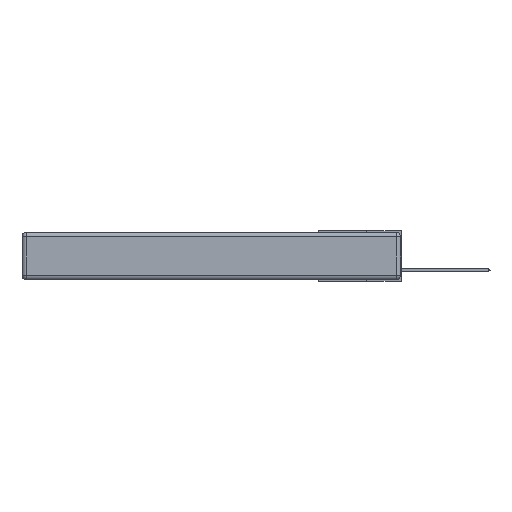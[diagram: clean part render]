
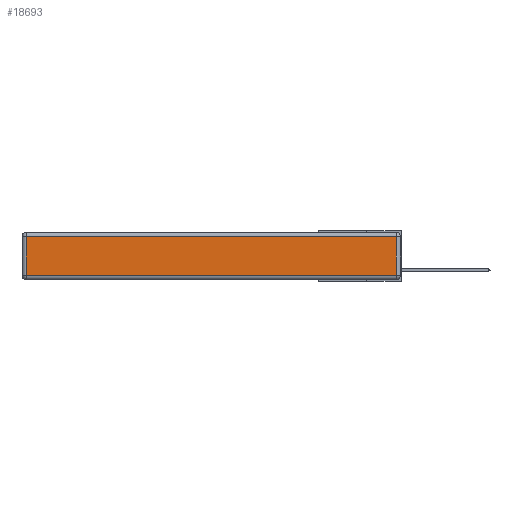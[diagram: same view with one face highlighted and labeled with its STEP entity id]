
A CAD part, left-side view. The second image highlights one B-rep face of the part: STEP entity #18693.
In plain terms, the highlighted planar face has unit normal (-1, 0, 0).
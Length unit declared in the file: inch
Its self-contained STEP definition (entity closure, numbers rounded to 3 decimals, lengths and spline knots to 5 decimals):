
#34 = LINE ( 'NONE', #2705, #7897 ) ;
#740 = DIRECTION ( 'NONE',  ( 0., -1., 0. ) ) ;
#1118 = ORIENTED_EDGE ( 'NONE', *, *, #17327, .T. ) ;
#1335 = EDGE_CURVE ( 'NONE', #22910, #4176, #34, .T. ) ;
#1951 = EDGE_LOOP ( 'NONE', ( #15078, #21452, #1118, #8721 ) ) ;
#2654 = CARTESIAN_POINT ( 'NONE',  ( 0., 0.03, -0.313 ) ) ;
#2705 = CARTESIAN_POINT ( 'NONE',  ( 0., 0.03, -0.343 ) ) ;
#4176 = VERTEX_POINT ( 'NONE', #23879 ) ;
#4275 = DIRECTION ( 'NONE',  ( 0., 0., -1. ) ) ;
#4941 = CARTESIAN_POINT ( 'NONE',  ( 0., 2.72, -0.313 ) ) ;
#6761 = VECTOR ( 'NONE', #740, 39.37008 ) ;
#7305 = VECTOR ( 'NONE', #4275, 39.37008 ) ;
#7897 = VECTOR ( 'NONE', #10509, 39.37008 ) ;
#8018 = LINE ( 'NONE', #22242, #24082 ) ;
#8721 = ORIENTED_EDGE ( 'NONE', *, *, #18146, .T. ) ;
#9157 = LINE ( 'NONE', #14294, #6761 ) ;
#9865 = CARTESIAN_POINT ( 'NONE',  ( 0., 0., -0.343 ) ) ;
#10509 = DIRECTION ( 'NONE',  ( 0., 0., 1. ) ) ;
#11072 = VERTEX_POINT ( 'NONE', #4941 ) ;
#11392 = VERTEX_POINT ( 'NONE', #21295 ) ;
#13704 = CARTESIAN_POINT ( 'NONE',  ( 0., 2.72, -0.343 ) ) ;
#14294 = CARTESIAN_POINT ( 'NONE',  ( 0., 0., -0.313 ) ) ;
#14467 = DIRECTION ( 'NONE',  ( 0., 1., 0. ) ) ;
#15078 = ORIENTED_EDGE ( 'NONE', *, *, #22888, .T. ) ;
#16198 = FACE_OUTER_BOUND ( 'NONE', #1951, .T. ) ;
#17327 = EDGE_CURVE ( 'NONE', #4176, #11392, #8018, .T. ) ;
#18034 = LINE ( 'NONE', #13704, #7305 ) ;
#18146 = EDGE_CURVE ( 'NONE', #11392, #11072, #18034, .T. ) ;
#18404 = AXIS2_PLACEMENT_3D ( 'NONE', #9865, #19324, #23289 ) ;
#18693 = ADVANCED_FACE ( 'NONE', ( #16198 ), #19650, .T. ) ;
#19324 = DIRECTION ( 'NONE',  ( -1., 0., 0. ) ) ;
#19650 = PLANE ( 'NONE',  #18404 ) ;
#21295 = CARTESIAN_POINT ( 'NONE',  ( 0., 2.72, -0.03 ) ) ;
#21452 = ORIENTED_EDGE ( 'NONE', *, *, #1335, .T. ) ;
#22242 = CARTESIAN_POINT ( 'NONE',  ( 0., 2.75, -0.03 ) ) ;
#22888 = EDGE_CURVE ( 'NONE', #11072, #22910, #9157, .T. ) ;
#22910 = VERTEX_POINT ( 'NONE', #2654 ) ;
#23289 = DIRECTION ( 'NONE',  ( 0., 0., 1. ) ) ;
#23879 = CARTESIAN_POINT ( 'NONE',  ( 0., 0.03, -0.03 ) ) ;
#24082 = VECTOR ( 'NONE', #14467, 39.37008 ) ;
